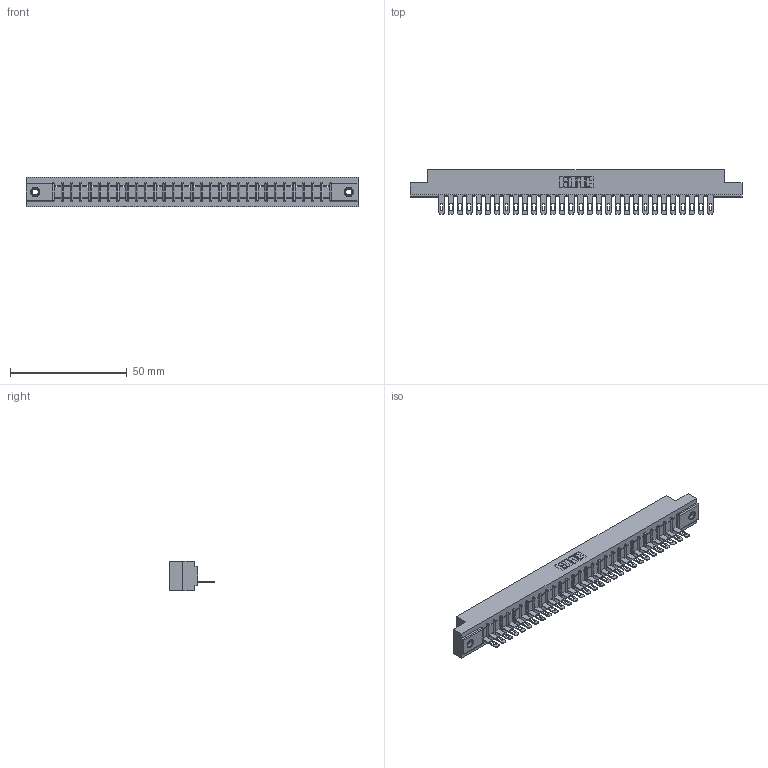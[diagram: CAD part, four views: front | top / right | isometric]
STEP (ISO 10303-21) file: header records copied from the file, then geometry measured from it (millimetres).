
FILE_DESCRIPTION (( 'STEP AP203' ), '1' );
FILE_NAME ('357-030-505-107.STEP', '2019-09-14T03:51:34', ( '' ), ( '' ), 'SwSTEP 2.0', 'SolidWorks 2016', '' );
FILE_SCHEMA (( 'CONFIG_CONTROL_DESIGN' ));
Length unit declared in the file: inch
Products named in the file (4): 307 Part_.156 Dia Mounting Holes; 357-030-505-107; 345-250-001_345-250-005-103; 307-290-001_505
Assembly tree (33 placements, depth 2):
  357-030-505-107
    307 Part_.156 Dia Mounting Holes
    307-290-001_505  x30
    345-250-001_345-250-005-103  x2
Bounding box: 141.88 x 19.18 x 12.7 mm (x, y, z)
Volume: 14688.1 mm3; surface area: 15699.2 mm2
Topology: 33 solids, 33 shells, 1889 faces, 5319 edges, 3414 vertices
Faces by surface type: plane 1182, cylinder 629, sphere 62, cone 12, torus 4
Entity records: 28357 total; most frequent: CARTESIAN_POINT 4751, ORIENTED_EDGE 4730, DIRECTION 4639, EDGE_CURVE 2365, LINE 1807, VECTOR 1807, VERTEX_POINT 1528, AXIS2_PLACEMENT_3D 1416
